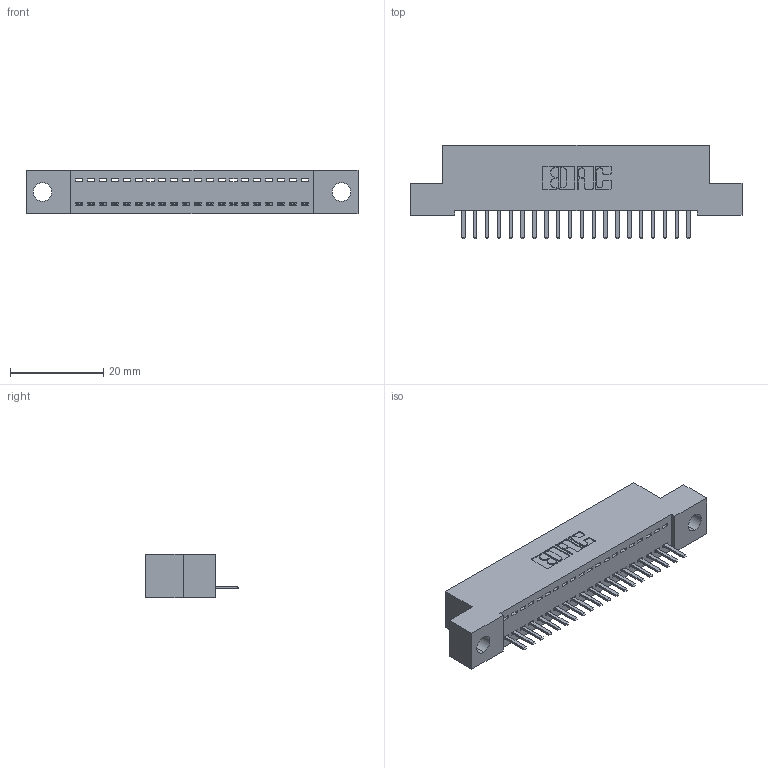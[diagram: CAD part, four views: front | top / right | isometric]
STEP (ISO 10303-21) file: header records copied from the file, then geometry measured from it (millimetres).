
FILE_DESCRIPTION (( 'STEP AP203' ), '1' );
FILE_NAME ('342-020-520-104.STEP', '2018-08-10T22:33:37', ( '' ), ( '' ), 'SwSTEP 2.0', 'SolidWorks 2016', '' );
FILE_SCHEMA (( 'CONFIG_CONTROL_DESIGN' ));
Length unit declared in the file: inch
Products named in the file (3): 342 Part_.156 TH; 345-292-001_345-293-120; 342-020-520-104
Assembly tree (21 placements, depth 2):
  342-020-520-104
    342 Part_.156 TH
    345-292-001_345-293-120  x20
Bounding box: 71.12 x 20.02 x 9.4 mm (x, y, z)
Volume: 6010.2 mm3; surface area: 8049.7 mm2
Topology: 21 solids, 21 shells, 1350 faces, 3979 edges, 2598 vertices
Faces by surface type: plane 946, cylinder 404
Entity records: 15057 total; most frequent: CARTESIAN_POINT 2618, ORIENTED_EDGE 2562, DIRECTION 2241, EDGE_CURVE 1281, LINE 1149, VECTOR 1149, VERTEX_POINT 850, AXIS2_PLACEMENT_3D 546
